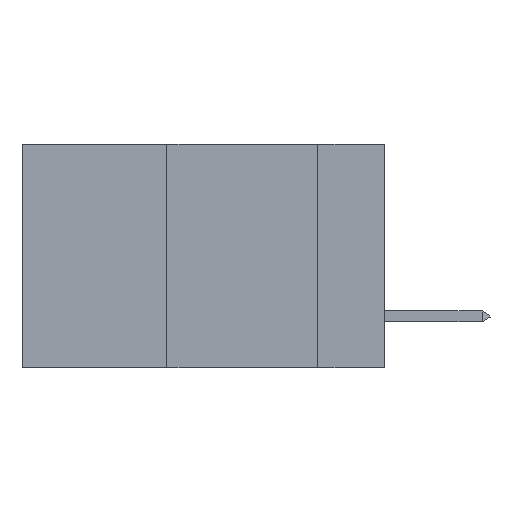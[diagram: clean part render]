
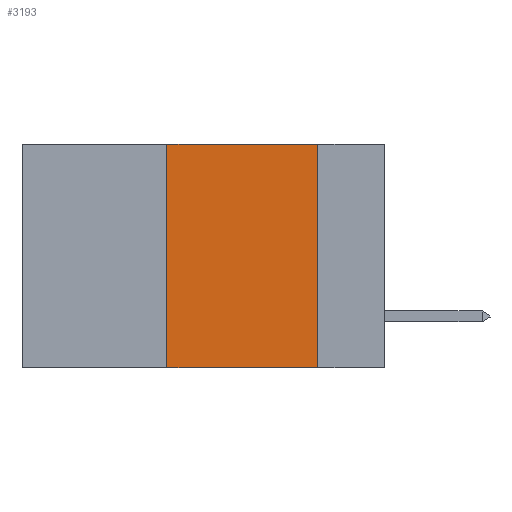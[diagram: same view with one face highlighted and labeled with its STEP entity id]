
A CAD part, left-side view. The second image highlights one B-rep face of the part: STEP entity #3193.
In plain terms, the highlighted planar face has unit normal (-1, 0, 0).
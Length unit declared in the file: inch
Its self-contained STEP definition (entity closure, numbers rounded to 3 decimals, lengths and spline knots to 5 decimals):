
#2149 = EDGE_CURVE ( 'NONE', #14755, #25046, #27942, .T. ) ;
#3193 = ADVANCED_FACE ( 'NONE', ( #14703 ), #18894, .F. ) ;
#4092 = LINE ( 'NONE', #6283, #25390 ) ;
#4161 = AXIS2_PLACEMENT_3D ( 'NONE', #36434, #4388, #33257 ) ;
#4388 = DIRECTION ( 'NONE',  ( 1., 0., 0. ) ) ;
#4400 = DIRECTION ( 'NONE',  ( 0., -1., 0. ) ) ;
#6283 = CARTESIAN_POINT ( 'NONE',  ( 0., 0.11, 0. ) ) ;
#8058 = VERTEX_POINT ( 'NONE', #36879 ) ;
#11453 = EDGE_CURVE ( 'NONE', #25046, #8058, #4092, .T. ) ;
#11581 = ORIENTED_EDGE ( 'NONE', *, *, #24276, .F. ) ;
#12601 = LINE ( 'NONE', #13665, #27568 ) ;
#12771 = EDGE_CURVE ( 'NONE', #34994, #8058, #25162, .T. ) ;
#13665 = CARTESIAN_POINT ( 'NONE',  ( 0., 0.36, 0. ) ) ;
#14703 = FACE_OUTER_BOUND ( 'NONE', #30432, .T. ) ;
#14755 = VERTEX_POINT ( 'NONE', #36374 ) ;
#15193 = ORIENTED_EDGE ( 'NONE', *, *, #12771, .T. ) ;
#16131 = CARTESIAN_POINT ( 'NONE',  ( 0., 0.6, 0. ) ) ;
#18894 = PLANE ( 'NONE',  #4161 ) ;
#20224 = VECTOR ( 'NONE', #4400, 39.37008 ) ;
#24276 = EDGE_CURVE ( 'NONE', #34994, #14755, #12601, .T. ) ;
#25046 = VERTEX_POINT ( 'NONE', #37221 ) ;
#25162 = LINE ( 'NONE', #33756, #30936 ) ;
#25390 = VECTOR ( 'NONE', #32251, 39.37008 ) ;
#27568 = VECTOR ( 'NONE', #36495, 39.37008 ) ;
#27942 = LINE ( 'NONE', #16131, #20224 ) ;
#28095 = CARTESIAN_POINT ( 'NONE',  ( 0., 0.36, -0.37 ) ) ;
#30432 = EDGE_LOOP ( 'NONE', ( #33642, #36744, #11581, #15193 ) ) ;
#30611 = DIRECTION ( 'NONE',  ( 0., -1., 0. ) ) ;
#30936 = VECTOR ( 'NONE', #30611, 39.37008 ) ;
#32251 = DIRECTION ( 'NONE',  ( 0., 0., -1. ) ) ;
#33257 = DIRECTION ( 'NONE',  ( 0., 0., -1. ) ) ;
#33642 = ORIENTED_EDGE ( 'NONE', *, *, #11453, .F. ) ;
#33756 = CARTESIAN_POINT ( 'NONE',  ( 0., 0.6, -0.37 ) ) ;
#34994 = VERTEX_POINT ( 'NONE', #28095 ) ;
#36374 = CARTESIAN_POINT ( 'NONE',  ( 0., 0.36, 0. ) ) ;
#36434 = CARTESIAN_POINT ( 'NONE',  ( 0., 0.6, 0. ) ) ;
#36495 = DIRECTION ( 'NONE',  ( 0., 0., 1. ) ) ;
#36744 = ORIENTED_EDGE ( 'NONE', *, *, #2149, .F. ) ;
#36879 = CARTESIAN_POINT ( 'NONE',  ( 0., 0.11, -0.37 ) ) ;
#37221 = CARTESIAN_POINT ( 'NONE',  ( 0., 0.11, 0. ) ) ;
